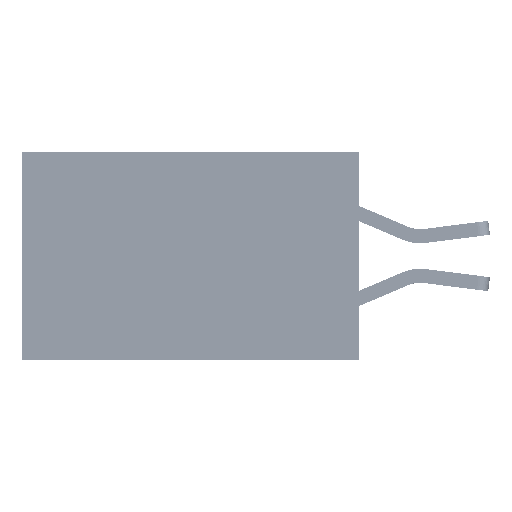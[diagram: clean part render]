
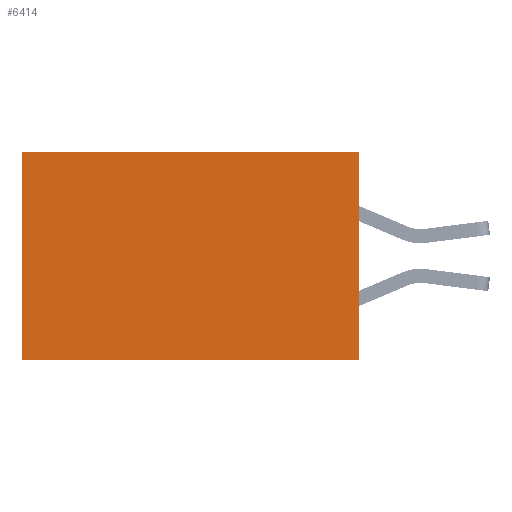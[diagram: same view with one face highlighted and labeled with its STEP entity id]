
A CAD part, left-side view. The second image highlights one B-rep face of the part: STEP entity #6414.
In plain terms, the highlighted planar face has unit normal (-1, 0, 0).
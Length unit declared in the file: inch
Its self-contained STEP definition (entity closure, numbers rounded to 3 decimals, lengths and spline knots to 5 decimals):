
#470 = EDGE_CURVE ( 'NONE', #14884, #15933, #7378, .T. ) ;
#2783 = ORIENTED_EDGE ( 'NONE', *, *, #28634, .T. ) ;
#3643 = CARTESIAN_POINT ( 'NONE',  ( 0.2875, 0.6, 0. ) ) ;
#5330 = EDGE_LOOP ( 'NONE', ( #2783, #21193, #35595, #32066 ) ) ;
#5877 = VECTOR ( 'NONE', #23987, 39.37008 ) ;
#6414 = ADVANCED_FACE ( 'NONE', ( #24033 ), #14100, .F. ) ;
#6491 = LINE ( 'NONE', #22711, #14502 ) ;
#7042 = AXIS2_PLACEMENT_3D ( 'NONE', #19975, #34989, #17107 ) ;
#7378 = LINE ( 'NONE', #18593, #30391 ) ;
#7719 = DIRECTION ( 'NONE',  ( 0., 0., -1. ) ) ;
#10814 = DIRECTION ( 'NONE',  ( 0., 1., 0. ) ) ;
#14100 = PLANE ( 'NONE',  #7042 ) ;
#14502 = VECTOR ( 'NONE', #7719, 39.37008 ) ;
#14884 = VERTEX_POINT ( 'NONE', #26924 ) ;
#15933 = VERTEX_POINT ( 'NONE', #3643 ) ;
#17107 = DIRECTION ( 'NONE',  ( 0., 0., -1. ) ) ;
#18562 = VERTEX_POINT ( 'NONE', #24545 ) ;
#18593 = CARTESIAN_POINT ( 'NONE',  ( 0.2875, 0., 0. ) ) ;
#19975 = CARTESIAN_POINT ( 'NONE',  ( 0.2875, 0., 0. ) ) ;
#20950 = CARTESIAN_POINT ( 'NONE',  ( 0.2875, 0.6, 0. ) ) ;
#21193 = ORIENTED_EDGE ( 'NONE', *, *, #24656, .F. ) ;
#22711 = CARTESIAN_POINT ( 'NONE',  ( 0.2875, 0., 0. ) ) ;
#23807 = CARTESIAN_POINT ( 'NONE',  ( 0.2875, 0.6, -0.37 ) ) ;
#23987 = DIRECTION ( 'NONE',  ( 0., 0., -1. ) ) ;
#24033 = FACE_OUTER_BOUND ( 'NONE', #5330, .T. ) ;
#24545 = CARTESIAN_POINT ( 'NONE',  ( 0.2875, 0., -0.37 ) ) ;
#24656 = EDGE_CURVE ( 'NONE', #18562, #26020, #35134, .T. ) ;
#25114 = DIRECTION ( 'NONE',  ( 0., 1., 0. ) ) ;
#26020 = VERTEX_POINT ( 'NONE', #23807 ) ;
#26295 = VECTOR ( 'NONE', #25114, 39.37008 ) ;
#26924 = CARTESIAN_POINT ( 'NONE',  ( 0.2875, 0., 0. ) ) ;
#26984 = EDGE_CURVE ( 'NONE', #14884, #18562, #6491, .T. ) ;
#28634 = EDGE_CURVE ( 'NONE', #15933, #26020, #28900, .T. ) ;
#28900 = LINE ( 'NONE', #20950, #5877 ) ;
#30391 = VECTOR ( 'NONE', #10814, 39.37008 ) ;
#32066 = ORIENTED_EDGE ( 'NONE', *, *, #470, .T. ) ;
#34093 = CARTESIAN_POINT ( 'NONE',  ( 0.2875, 0., -0.37 ) ) ;
#34989 = DIRECTION ( 'NONE',  ( 1., 0., 0. ) ) ;
#35134 = LINE ( 'NONE', #34093, #26295 ) ;
#35595 = ORIENTED_EDGE ( 'NONE', *, *, #26984, .F. ) ;
